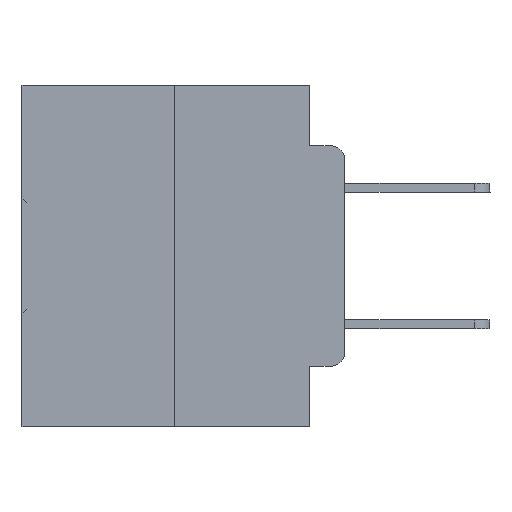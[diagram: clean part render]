
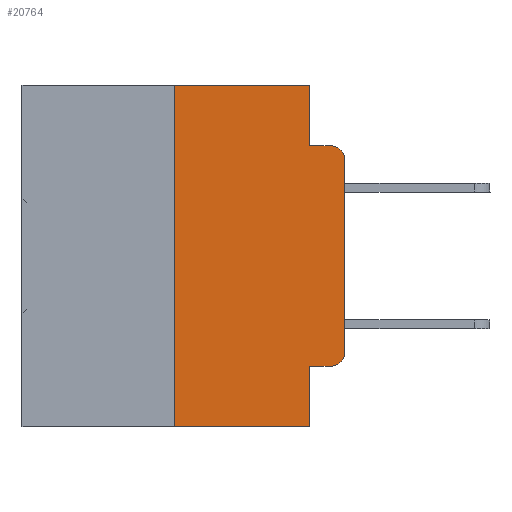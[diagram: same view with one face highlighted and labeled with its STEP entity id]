
A CAD part, left-side view. The second image highlights one B-rep face of the part: STEP entity #20764.
In plain terms, the highlighted planar face has unit normal (-1, 0, 0).
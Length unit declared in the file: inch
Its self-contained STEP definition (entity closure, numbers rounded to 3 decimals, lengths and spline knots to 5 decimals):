
#272 = CARTESIAN_POINT ( 'NONE',  ( 0., 0.051, -0.0885 ) ) ;
#292 = DIRECTION ( 'NONE',  ( 0., 0., -1. ) ) ;
#950 = VERTEX_POINT ( 'NONE', #21366 ) ;
#1328 = ORIENTED_EDGE ( 'NONE', *, *, #18861, .F. ) ;
#1509 = LINE ( 'NONE', #18479, #28881 ) ;
#1941 = VERTEX_POINT ( 'NONE', #15181 ) ;
#2268 = EDGE_CURVE ( 'NONE', #16479, #950, #28347, .T. ) ;
#2545 = LINE ( 'NONE', #32747, #15963 ) ;
#3176 = EDGE_CURVE ( 'NONE', #27725, #9770, #2545, .T. ) ;
#3853 = DIRECTION ( 'NONE',  ( 0., -1., 0. ) ) ;
#4365 = EDGE_CURVE ( 'NONE', #9770, #9298, #26133, .T. ) ;
#4835 = CARTESIAN_POINT ( 'NONE',  ( 0., 0.02, -0.3915 ) ) ;
#5040 = ORIENTED_EDGE ( 'NONE', *, *, #4365, .F. ) ;
#5708 = CARTESIAN_POINT ( 'NONE',  ( 0., 0.25, 0. ) ) ;
#6308 = VECTOR ( 'NONE', #29069, 39.37008 ) ;
#6735 = LINE ( 'NONE', #11992, #20986 ) ;
#7778 = DIRECTION ( 'NONE',  ( 0., 0., 1. ) ) ;
#7904 = DIRECTION ( 'NONE',  ( 0., -1., 0. ) ) ;
#8390 = ORIENTED_EDGE ( 'NONE', *, *, #9921, .T. ) ;
#9203 = DIRECTION ( 'NONE',  ( 0., 0., 1. ) ) ;
#9286 = VERTEX_POINT ( 'NONE', #26758 ) ;
#9298 = VERTEX_POINT ( 'NONE', #272 ) ;
#9770 = VERTEX_POINT ( 'NONE', #33791 ) ;
#9875 = AXIS2_PLACEMENT_3D ( 'NONE', #4835, #18529, #18803 ) ;
#9921 = EDGE_CURVE ( 'NONE', #9286, #16479, #25154, .T. ) ;
#10413 = CARTESIAN_POINT ( 'NONE',  ( 0., 0.02, -0.0885 ) ) ;
#10544 = LINE ( 'NONE', #22332, #16810 ) ;
#10548 = ORIENTED_EDGE ( 'NONE', *, *, #28402, .F. ) ;
#11159 = CARTESIAN_POINT ( 'NONE',  ( 0., 0.25, -0.5 ) ) ;
#11675 = DIRECTION ( 'NONE',  ( 0., -1., 0. ) ) ;
#11992 = CARTESIAN_POINT ( 'NONE',  ( 0., 0.051, -0.0885 ) ) ;
#12144 = VECTOR ( 'NONE', #26266, 39.37008 ) ;
#13189 = EDGE_CURVE ( 'NONE', #1941, #29998, #13244, .T. ) ;
#13244 = CIRCLE ( 'NONE', #21236, 0.02 ) ;
#13484 = DIRECTION ( 'NONE',  ( 0., 0., -1. ) ) ;
#13520 = LINE ( 'NONE', #18558, #6308 ) ;
#14621 = VERTEX_POINT ( 'NONE', #23644 ) ;
#15181 = CARTESIAN_POINT ( 'NONE',  ( 0., 0., -0.1085 ) ) ;
#15963 = VECTOR ( 'NONE', #32439, 39.37008 ) ;
#16035 = PLANE ( 'NONE',  #17107 ) ;
#16357 = DIRECTION ( 'NONE',  ( -1., 0., 0. ) ) ;
#16479 = VERTEX_POINT ( 'NONE', #21044 ) ;
#16810 = VECTOR ( 'NONE', #11675, 39.37008 ) ;
#17107 = AXIS2_PLACEMENT_3D ( 'NONE', #21352, #29215, #13484 ) ;
#17201 = CARTESIAN_POINT ( 'NONE',  ( 0., 0.25, 0. ) ) ;
#17695 = CARTESIAN_POINT ( 'NONE',  ( 0., 0.051, 0. ) ) ;
#18080 = ORIENTED_EDGE ( 'NONE', *, *, #2268, .T. ) ;
#18191 = VECTOR ( 'NONE', #7904, 39.37008 ) ;
#18319 = VERTEX_POINT ( 'NONE', #11159 ) ;
#18479 = CARTESIAN_POINT ( 'NONE',  ( 0., 0., 0. ) ) ;
#18529 = DIRECTION ( 'NONE',  ( -1., 0., 0. ) ) ;
#18558 = CARTESIAN_POINT ( 'NONE',  ( 0., 0.051, 0. ) ) ;
#18803 = DIRECTION ( 'NONE',  ( 0., 0., -1. ) ) ;
#18861 = EDGE_CURVE ( 'NONE', #9286, #14621, #13520, .T. ) ;
#19293 = ORIENTED_EDGE ( 'NONE', *, *, #3176, .F. ) ;
#19895 = LINE ( 'NONE', #17201, #25998 ) ;
#20546 = ORIENTED_EDGE ( 'NONE', *, *, #22501, .T. ) ;
#20764 = ADVANCED_FACE ( 'NONE', ( #27365 ), #16035, .F. ) ;
#20959 = ORIENTED_EDGE ( 'NONE', *, *, #32233, .F. ) ;
#20986 = VECTOR ( 'NONE', #3853, 39.37008 ) ;
#21044 = CARTESIAN_POINT ( 'NONE',  ( 0., 0.02, -0.4115 ) ) ;
#21236 = AXIS2_PLACEMENT_3D ( 'NONE', #32032, #16357, #292 ) ;
#21253 = CARTESIAN_POINT ( 'NONE',  ( 0., 0.051, -0.4115 ) ) ;
#21352 = CARTESIAN_POINT ( 'NONE',  ( 0., 0.473, 0. ) ) ;
#21366 = CARTESIAN_POINT ( 'NONE',  ( 0., 0., -0.3915 ) ) ;
#21778 = ORIENTED_EDGE ( 'NONE', *, *, #28957, .T. ) ;
#22332 = CARTESIAN_POINT ( 'NONE',  ( 0., 0.473, -0.5 ) ) ;
#22501 = EDGE_CURVE ( 'NONE', #950, #1941, #1509, .T. ) ;
#23644 = CARTESIAN_POINT ( 'NONE',  ( 0., 0.051, -0.5 ) ) ;
#25154 = LINE ( 'NONE', #21253, #18191 ) ;
#25998 = VECTOR ( 'NONE', #9203, 39.37008 ) ;
#26133 = LINE ( 'NONE', #17695, #12144 ) ;
#26266 = DIRECTION ( 'NONE',  ( 0., 0., -1. ) ) ;
#26758 = CARTESIAN_POINT ( 'NONE',  ( 0., 0.051, -0.4115 ) ) ;
#27365 = FACE_OUTER_BOUND ( 'NONE', #30155, .T. ) ;
#27725 = VERTEX_POINT ( 'NONE', #5708 ) ;
#28347 = CIRCLE ( 'NONE', #9875, 0.02 ) ;
#28402 = EDGE_CURVE ( 'NONE', #9298, #29998, #6735, .T. ) ;
#28881 = VECTOR ( 'NONE', #7778, 39.37008 ) ;
#28957 = EDGE_CURVE ( 'NONE', #18319, #14621, #10544, .T. ) ;
#29069 = DIRECTION ( 'NONE',  ( 0., 0., -1. ) ) ;
#29092 = ORIENTED_EDGE ( 'NONE', *, *, #13189, .T. ) ;
#29215 = DIRECTION ( 'NONE',  ( 1., 0., 0. ) ) ;
#29998 = VERTEX_POINT ( 'NONE', #10413 ) ;
#30155 = EDGE_LOOP ( 'NONE', ( #20546, #29092, #10548, #5040, #19293, #20959, #21778, #1328, #8390, #18080 ) ) ;
#32032 = CARTESIAN_POINT ( 'NONE',  ( 0., 0.02, -0.1085 ) ) ;
#32233 = EDGE_CURVE ( 'NONE', #18319, #27725, #19895, .T. ) ;
#32439 = DIRECTION ( 'NONE',  ( 0., -1., 0. ) ) ;
#32747 = CARTESIAN_POINT ( 'NONE',  ( 0., 0.473, 0. ) ) ;
#33791 = CARTESIAN_POINT ( 'NONE',  ( 0., 0.051, 0. ) ) ;
